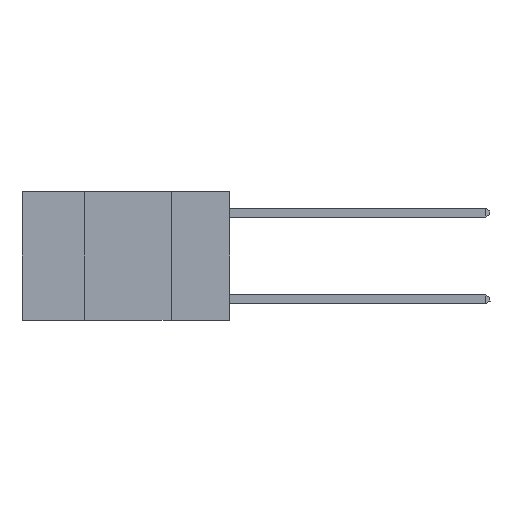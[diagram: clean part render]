
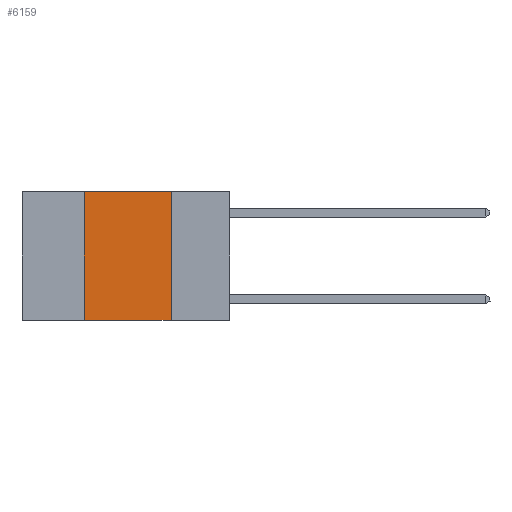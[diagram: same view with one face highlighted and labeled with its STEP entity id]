
A CAD part, left-side view. The second image highlights one B-rep face of the part: STEP entity #6159.
In plain terms, the highlighted planar face has unit normal (-1, 0, 0).
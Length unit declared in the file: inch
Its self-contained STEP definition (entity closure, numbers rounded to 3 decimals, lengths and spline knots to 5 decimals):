
#1585 = CARTESIAN_POINT ( 'NONE',  ( 0., 0.42, 0. ) ) ;
#3304 = VECTOR ( 'NONE', #10148, 39.37008 ) ;
#3685 = CARTESIAN_POINT ( 'NONE',  ( 0., 0.17, -0.37 ) ) ;
#3809 = VERTEX_POINT ( 'NONE', #23392 ) ;
#4076 = EDGE_CURVE ( 'NONE', #3809, #4218, #26402, .T. ) ;
#4218 = VERTEX_POINT ( 'NONE', #1585 ) ;
#4316 = ORIENTED_EDGE ( 'NONE', *, *, #21406, .F. ) ;
#4938 = CARTESIAN_POINT ( 'NONE',  ( 0., 0.42, 0. ) ) ;
#6159 = ADVANCED_FACE ( 'NONE', ( #16734 ), #19203, .F. ) ;
#8169 = EDGE_LOOP ( 'NONE', ( #4316, #21033, #22915, #8839 ) ) ;
#8337 = DIRECTION ( 'NONE',  ( 0., 0., -1. ) ) ;
#8839 = ORIENTED_EDGE ( 'NONE', *, *, #15922, .T. ) ;
#10119 = LINE ( 'NONE', #26772, #20073 ) ;
#10148 = DIRECTION ( 'NONE',  ( 0., -1., 0. ) ) ;
#11278 = VECTOR ( 'NONE', #15958, 39.37008 ) ;
#12212 = CARTESIAN_POINT ( 'NONE',  ( 0., 0.6, 0. ) ) ;
#13063 = LINE ( 'NONE', #17058, #17312 ) ;
#13744 = CARTESIAN_POINT ( 'NONE',  ( 0., 0.17, 0. ) ) ;
#15922 = EDGE_CURVE ( 'NONE', #3809, #24033, #13063, .T. ) ;
#15958 = DIRECTION ( 'NONE',  ( 0., 0., 1. ) ) ;
#16734 = FACE_OUTER_BOUND ( 'NONE', #8169, .T. ) ;
#16899 = VERTEX_POINT ( 'NONE', #13744 ) ;
#17058 = CARTESIAN_POINT ( 'NONE',  ( 0., 0.6, -0.37 ) ) ;
#17312 = VECTOR ( 'NONE', #25712, 39.37008 ) ;
#18523 = EDGE_CURVE ( 'NONE', #4218, #16899, #26943, .T. ) ;
#19066 = DIRECTION ( 'NONE',  ( 1., 0., 0. ) ) ;
#19203 = PLANE ( 'NONE',  #20713 ) ;
#19471 = CARTESIAN_POINT ( 'NONE',  ( 0., 0.6, 0. ) ) ;
#20073 = VECTOR ( 'NONE', #20581, 39.37008 ) ;
#20581 = DIRECTION ( 'NONE',  ( 0., 0., -1. ) ) ;
#20713 = AXIS2_PLACEMENT_3D ( 'NONE', #19471, #19066, #8337 ) ;
#21033 = ORIENTED_EDGE ( 'NONE', *, *, #18523, .F. ) ;
#21406 = EDGE_CURVE ( 'NONE', #16899, #24033, #10119, .T. ) ;
#22915 = ORIENTED_EDGE ( 'NONE', *, *, #4076, .F. ) ;
#23392 = CARTESIAN_POINT ( 'NONE',  ( 0., 0.42, -0.37 ) ) ;
#24033 = VERTEX_POINT ( 'NONE', #3685 ) ;
#25712 = DIRECTION ( 'NONE',  ( 0., -1., 0. ) ) ;
#26402 = LINE ( 'NONE', #4938, #11278 ) ;
#26772 = CARTESIAN_POINT ( 'NONE',  ( 0., 0.17, 0. ) ) ;
#26943 = LINE ( 'NONE', #12212, #3304 ) ;
